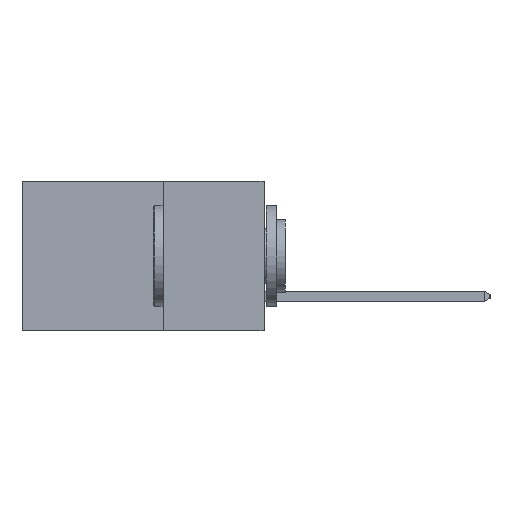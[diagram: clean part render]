
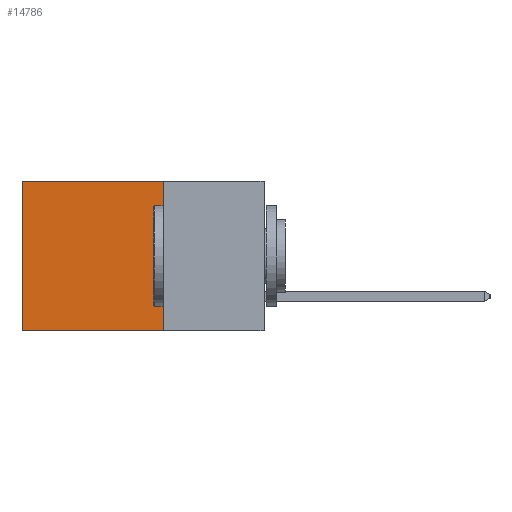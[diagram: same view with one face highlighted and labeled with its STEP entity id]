
A CAD part, left-side view. The second image highlights one B-rep face of the part: STEP entity #14786.
In plain terms, the highlighted planar face has unit normal (-1, 0, 0).
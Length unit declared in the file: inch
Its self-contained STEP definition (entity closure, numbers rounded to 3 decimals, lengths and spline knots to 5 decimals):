
#532 = LINE ( 'NONE', #6125, #10211 ) ;
#801 = PLANE ( 'NONE',  #8150 ) ;
#1947 = LINE ( 'NONE', #7698, #4819 ) ;
#2058 = DIRECTION ( 'NONE',  ( 1., 0., 0. ) ) ;
#2868 = ORIENTED_EDGE ( 'NONE', *, *, #15167, .T. ) ;
#3057 = CARTESIAN_POINT ( 'NONE',  ( 0.2615, 0.25, 0. ) ) ;
#4677 = CARTESIAN_POINT ( 'NONE',  ( 0.2615, 0.25, -0.37 ) ) ;
#4780 = LINE ( 'NONE', #6882, #8378 ) ;
#4819 = VECTOR ( 'NONE', #5238, 39.37008 ) ;
#4936 = EDGE_CURVE ( 'NONE', #5827, #10916, #4780, .T. ) ;
#5238 = DIRECTION ( 'NONE',  ( 0., 1., 0. ) ) ;
#5239 = CARTESIAN_POINT ( 'NONE',  ( 0.2615, 0.25, -0.37 ) ) ;
#5528 = CARTESIAN_POINT ( 'NONE',  ( 0.2615, 0.6, -0.37 ) ) ;
#5827 = VERTEX_POINT ( 'NONE', #7480 ) ;
#6125 = CARTESIAN_POINT ( 'NONE',  ( 0.2615, 0.25, -0.37 ) ) ;
#6391 = VECTOR ( 'NONE', #10698, 39.37008 ) ;
#6882 = CARTESIAN_POINT ( 'NONE',  ( 0.2615, 0.6, -0.37 ) ) ;
#6906 = DIRECTION ( 'NONE',  ( 0., 0., -1. ) ) ;
#6926 = CARTESIAN_POINT ( 'NONE',  ( 0.2615, 0.25, -0.37 ) ) ;
#7064 = EDGE_CURVE ( 'NONE', #9457, #10916, #532, .T. ) ;
#7266 = VERTEX_POINT ( 'NONE', #3057 ) ;
#7480 = CARTESIAN_POINT ( 'NONE',  ( 0.2615, 0.6, 0. ) ) ;
#7698 = CARTESIAN_POINT ( 'NONE',  ( 0.2615, 0.25, 0. ) ) ;
#8150 = AXIS2_PLACEMENT_3D ( 'NONE', #6926, #2058, #10555 ) ;
#8378 = VECTOR ( 'NONE', #6906, 39.37008 ) ;
#8527 = ORIENTED_EDGE ( 'NONE', *, *, #4936, .T. ) ;
#9457 = VERTEX_POINT ( 'NONE', #5239 ) ;
#10211 = VECTOR ( 'NONE', #13127, 39.37008 ) ;
#10555 = DIRECTION ( 'NONE',  ( 0., 0., -1. ) ) ;
#10698 = DIRECTION ( 'NONE',  ( 0., 0., -1. ) ) ;
#10862 = FACE_OUTER_BOUND ( 'NONE', #14368, .T. ) ;
#10916 = VERTEX_POINT ( 'NONE', #5528 ) ;
#11866 = ORIENTED_EDGE ( 'NONE', *, *, #7064, .F. ) ;
#12271 = LINE ( 'NONE', #4677, #6391 ) ;
#13127 = DIRECTION ( 'NONE',  ( 0., 1., 0. ) ) ;
#14292 = EDGE_CURVE ( 'NONE', #7266, #9457, #12271, .T. ) ;
#14368 = EDGE_LOOP ( 'NONE', ( #8527, #11866, #15255, #2868 ) ) ;
#14786 = ADVANCED_FACE ( 'NONE', ( #10862 ), #801, .F. ) ;
#15167 = EDGE_CURVE ( 'NONE', #7266, #5827, #1947, .T. ) ;
#15255 = ORIENTED_EDGE ( 'NONE', *, *, #14292, .F. ) ;
